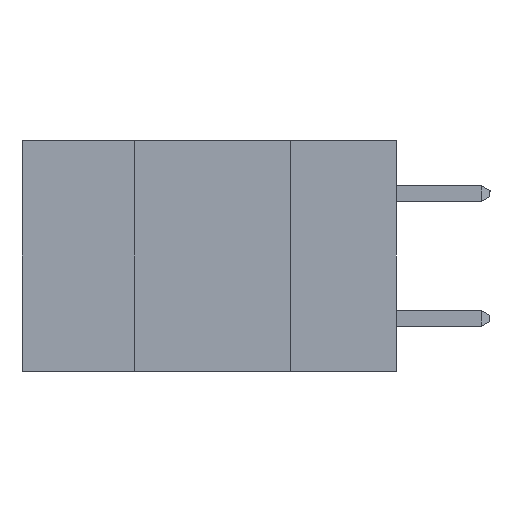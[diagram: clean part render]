
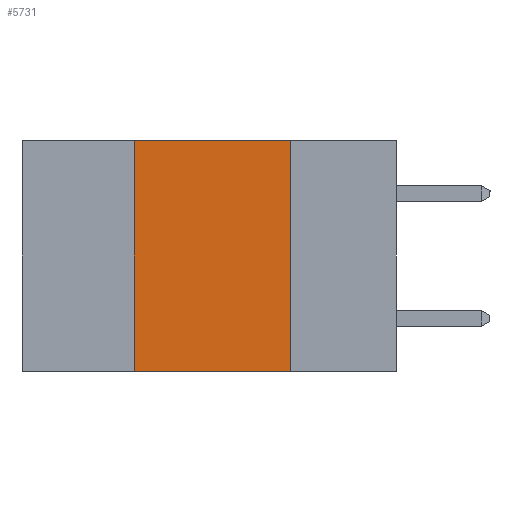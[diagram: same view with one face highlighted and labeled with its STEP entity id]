
A CAD part, left-side view. The second image highlights one B-rep face of the part: STEP entity #5731.
In plain terms, the highlighted planar face has unit normal (-1, 0, 0).
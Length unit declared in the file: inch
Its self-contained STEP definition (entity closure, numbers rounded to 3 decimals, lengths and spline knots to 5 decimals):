
#670 = AXIS2_PLACEMENT_3D ( 'NONE', #1045, #988, #9516 ) ;
#988 = DIRECTION ( 'NONE',  ( 1., 0., 0. ) ) ;
#1045 = CARTESIAN_POINT ( 'NONE',  ( 0., 0.6, 0. ) ) ;
#2059 = LINE ( 'NONE', #3994, #2228 ) ;
#2228 = VECTOR ( 'NONE', #3794, 39.37008 ) ;
#2247 = EDGE_CURVE ( 'NONE', #9371, #5492, #7438, .T. ) ;
#2838 = VECTOR ( 'NONE', #7269, 39.37008 ) ;
#3238 = VECTOR ( 'NONE', #5274, 39.37008 ) ;
#3534 = CARTESIAN_POINT ( 'NONE',  ( 0., 0.17, -0.37 ) ) ;
#3794 = DIRECTION ( 'NONE',  ( 0., 0., -1. ) ) ;
#3994 = CARTESIAN_POINT ( 'NONE',  ( 0., 0.17, -0.37 ) ) ;
#4463 = DIRECTION ( 'NONE',  ( 0., 0., 1. ) ) ;
#4533 = CARTESIAN_POINT ( 'NONE',  ( 0., 0.42, -0.37 ) ) ;
#4719 = FACE_OUTER_BOUND ( 'NONE', #5602, .T. ) ;
#4743 = ORIENTED_EDGE ( 'NONE', *, *, #4901, .F. ) ;
#4901 = EDGE_CURVE ( 'NONE', #4926, #6864, #2059, .T. ) ;
#4926 = VERTEX_POINT ( 'NONE', #7341 ) ;
#5274 = DIRECTION ( 'NONE',  ( 0., -1., 0. ) ) ;
#5293 = CARTESIAN_POINT ( 'NONE',  ( 0., 0.6, 0. ) ) ;
#5492 = VERTEX_POINT ( 'NONE', #9719 ) ;
#5536 = LINE ( 'NONE', #5293, #2838 ) ;
#5602 = EDGE_LOOP ( 'NONE', ( #4743, #6814, #11788, #9370 ) ) ;
#5635 = EDGE_CURVE ( 'NONE', #5492, #4926, #5536, .T. ) ;
#5731 = ADVANCED_FACE ( 'NONE', ( #4719 ), #9570, .F. ) ;
#6107 = EDGE_CURVE ( 'NONE', #9371, #6864, #6198, .T. ) ;
#6198 = LINE ( 'NONE', #8066, #3238 ) ;
#6814 = ORIENTED_EDGE ( 'NONE', *, *, #5635, .F. ) ;
#6864 = VERTEX_POINT ( 'NONE', #3534 ) ;
#7269 = DIRECTION ( 'NONE',  ( 0., -1., 0. ) ) ;
#7341 = CARTESIAN_POINT ( 'NONE',  ( 0., 0.17, 0. ) ) ;
#7438 = LINE ( 'NONE', #4533, #8728 ) ;
#8066 = CARTESIAN_POINT ( 'NONE',  ( 0., 0.6, -0.37 ) ) ;
#8728 = VECTOR ( 'NONE', #4463, 39.37008 ) ;
#9370 = ORIENTED_EDGE ( 'NONE', *, *, #6107, .T. ) ;
#9371 = VERTEX_POINT ( 'NONE', #11750 ) ;
#9516 = DIRECTION ( 'NONE',  ( 0., 0., -1. ) ) ;
#9570 = PLANE ( 'NONE',  #670 ) ;
#9719 = CARTESIAN_POINT ( 'NONE',  ( 0., 0.42, 0. ) ) ;
#11750 = CARTESIAN_POINT ( 'NONE',  ( 0., 0.42, -0.37 ) ) ;
#11788 = ORIENTED_EDGE ( 'NONE', *, *, #2247, .F. ) ;
